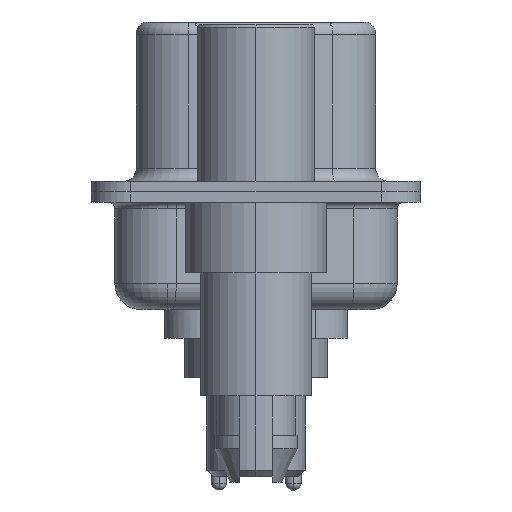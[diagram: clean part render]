
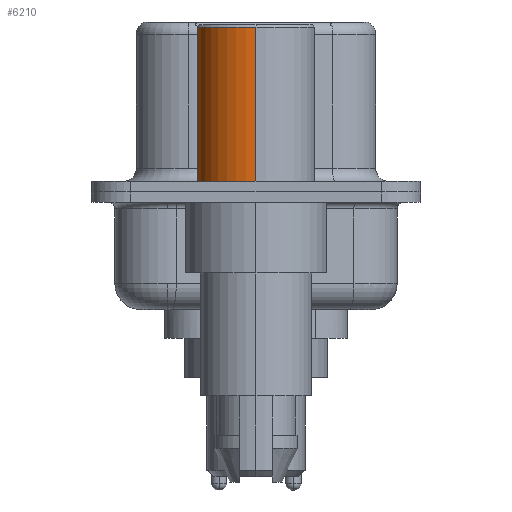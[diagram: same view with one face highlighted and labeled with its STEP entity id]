
A CAD part, left-side view. The second image highlights one B-rep face of the part: STEP entity #6210.
In plain terms, the highlighted cylindrical face has radius 2.25 mm (diameter 4.5 mm), a partial arc.
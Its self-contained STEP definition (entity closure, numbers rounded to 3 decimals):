
#577 = CARTESIAN_POINT ( 'NONE',  ( 0., 0., 0.4 ) ) ;
#692 = LINE ( 'NONE', #2323, #12291 ) ;
#1042 = DIRECTION ( 'NONE',  ( 0., 0., 1. ) ) ;
#1114 = ORIENTED_EDGE ( 'NONE', *, *, #16386, .T. ) ;
#1171 = DIRECTION ( 'NONE',  ( 1., 0., 0. ) ) ;
#1273 = CARTESIAN_POINT ( 'NONE',  ( -2.25, 0., 6.3 ) ) ;
#1388 = CARTESIAN_POINT ( 'NONE',  ( -2.25, 0., 0.581 ) ) ;
#2116 = DIRECTION ( 'NONE',  ( 0., 0., 1. ) ) ;
#2131 = DIRECTION ( 'NONE',  ( 1., 0., 0. ) ) ;
#2294 = DIRECTION ( 'NONE',  ( 0., 0., 1. ) ) ;
#2323 = CARTESIAN_POINT ( 'NONE',  ( 2.25, 0., 0.581 ) ) ;
#2617 = ORIENTED_EDGE ( 'NONE', *, *, #11520, .F. ) ;
#3283 = LINE ( 'NONE', #1388, #18828 ) ;
#6210 = ADVANCED_FACE ( 'NONE', ( #19590 ), #10653, .T. ) ;
#6286 = ORIENTED_EDGE ( 'NONE', *, *, #7343, .T. ) ;
#6342 = EDGE_CURVE ( 'NONE', #18529, #6362, #692, .T. ) ;
#6362 = VERTEX_POINT ( 'NONE', #9802 ) ;
#6386 = CIRCLE ( 'NONE', #12503, 2.25 ) ;
#6477 = AXIS2_PLACEMENT_3D ( 'NONE', #577, #11183, #2131 ) ;
#7343 = EDGE_CURVE ( 'NONE', #16726, #8739, #3283, .T. ) ;
#8556 = DIRECTION ( 'NONE',  ( 0., 0., 1. ) ) ;
#8618 = CARTESIAN_POINT ( 'NONE',  ( 2.25, 0., 0.4 ) ) ;
#8660 = ORIENTED_EDGE ( 'NONE', *, *, #6342, .F. ) ;
#8739 = VERTEX_POINT ( 'NONE', #1273 ) ;
#9802 = CARTESIAN_POINT ( 'NONE',  ( 2.25, 0., 6.3 ) ) ;
#10653 = CYLINDRICAL_SURFACE ( 'NONE', #11312, 2.25 ) ;
#11183 = DIRECTION ( 'NONE',  ( 0., 0., 1. ) ) ;
#11312 = AXIS2_PLACEMENT_3D ( 'NONE', #15618, #2116, #1171 ) ;
#11520 = EDGE_CURVE ( 'NONE', #6362, #8739, #6386, .T. ) ;
#11855 = CIRCLE ( 'NONE', #6477, 2.25 ) ;
#12291 = VECTOR ( 'NONE', #2294, 1000. ) ;
#12503 = AXIS2_PLACEMENT_3D ( 'NONE', #17637, #8556, #19188 ) ;
#14629 = EDGE_LOOP ( 'NONE', ( #1114, #6286, #2617, #8660 ) ) ;
#14959 = CARTESIAN_POINT ( 'NONE',  ( -2.25, 0., 0.4 ) ) ;
#15618 = CARTESIAN_POINT ( 'NONE',  ( 0., 0., 0.581 ) ) ;
#16386 = EDGE_CURVE ( 'NONE', #18529, #16726, #11855, .T. ) ;
#16726 = VERTEX_POINT ( 'NONE', #14959 ) ;
#17637 = CARTESIAN_POINT ( 'NONE',  ( 0., 0., 6.3 ) ) ;
#18529 = VERTEX_POINT ( 'NONE', #8618 ) ;
#18828 = VECTOR ( 'NONE', #1042, 1000. ) ;
#19188 = DIRECTION ( 'NONE',  ( 1., 0., 0. ) ) ;
#19590 = FACE_OUTER_BOUND ( 'NONE', #14629, .T. ) ;
